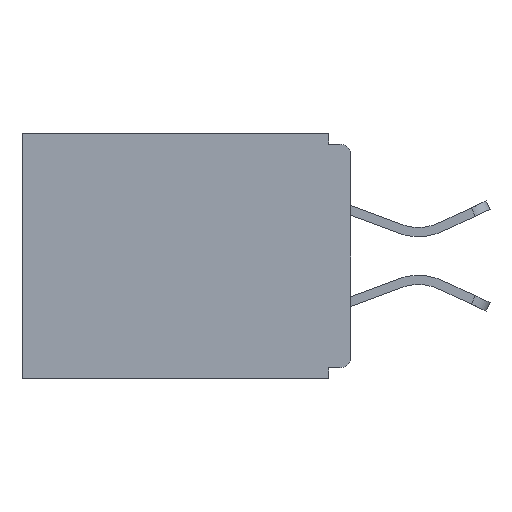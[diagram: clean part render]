
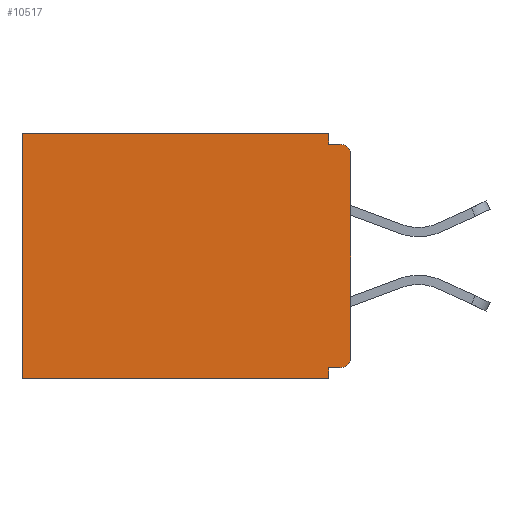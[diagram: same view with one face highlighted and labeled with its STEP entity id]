
A CAD part, left-side view. The second image highlights one B-rep face of the part: STEP entity #10517.
In plain terms, the highlighted planar face has unit normal (-1, 0, 0).
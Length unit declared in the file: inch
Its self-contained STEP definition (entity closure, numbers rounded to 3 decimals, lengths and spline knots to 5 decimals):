
#258 = ORIENTED_EDGE ( 'NONE', *, *, #4123, .F. ) ;
#387 = VERTEX_POINT ( 'NONE', #2516 ) ;
#434 = EDGE_CURVE ( 'NONE', #1373, #4286, #1137, .T. ) ;
#645 = DIRECTION ( 'NONE',  ( 0., 0., -1. ) ) ;
#848 = ORIENTED_EDGE ( 'NONE', *, *, #3834, .T. ) ;
#878 = CARTESIAN_POINT ( 'NONE',  ( 0.298, 0.015, -0.015 ) ) ;
#886 = VERTEX_POINT ( 'NONE', #5355 ) ;
#1010 = VECTOR ( 'NONE', #9738, 39.37008 ) ;
#1051 = ORIENTED_EDGE ( 'NONE', *, *, #8999, .T. ) ;
#1137 = LINE ( 'NONE', #3594, #8095 ) ;
#1141 = EDGE_CURVE ( 'NONE', #886, #8241, #9219, .T. ) ;
#1291 = LINE ( 'NONE', #1672, #3971 ) ;
#1373 = VERTEX_POINT ( 'NONE', #10183 ) ;
#1511 = CARTESIAN_POINT ( 'NONE',  ( 0.298, 0.031, -0.343 ) ) ;
#1668 = CARTESIAN_POINT ( 'NONE',  ( 0.298, 0.46, 0. ) ) ;
#1672 = CARTESIAN_POINT ( 'NONE',  ( 0.298, 0., -0.328 ) ) ;
#2212 = EDGE_CURVE ( 'NONE', #10403, #3517, #7458, .T. ) ;
#2218 = DIRECTION ( 'NONE',  ( 1., 0., 0. ) ) ;
#2272 = VERTEX_POINT ( 'NONE', #9874 ) ;
#2301 = LINE ( 'NONE', #1511, #4550 ) ;
#2417 = DIRECTION ( 'NONE',  ( 0., 1., 0. ) ) ;
#2439 = LINE ( 'NONE', #2885, #3441 ) ;
#2495 = CARTESIAN_POINT ( 'NONE',  ( 0.298, 0., 0. ) ) ;
#2516 = CARTESIAN_POINT ( 'NONE',  ( 0.298, 0.031, 0. ) ) ;
#2550 = CIRCLE ( 'NONE', #5939, 0.015 ) ;
#2885 = CARTESIAN_POINT ( 'NONE',  ( 0.298, 0.46, 0. ) ) ;
#3245 = CARTESIAN_POINT ( 'NONE',  ( 0.298, 0., 0. ) ) ;
#3380 = VECTOR ( 'NONE', #7256, 39.37008 ) ;
#3441 = VECTOR ( 'NONE', #6486, 39.37008 ) ;
#3517 = VERTEX_POINT ( 'NONE', #878 ) ;
#3594 = CARTESIAN_POINT ( 'NONE',  ( 0.298, 0., -0.343 ) ) ;
#3688 = ORIENTED_EDGE ( 'NONE', *, *, #434, .F. ) ;
#3762 = CARTESIAN_POINT ( 'NONE',  ( 0.298, 0.015, -0.328 ) ) ;
#3834 = EDGE_CURVE ( 'NONE', #7170, #4286, #2439, .T. ) ;
#3971 = VECTOR ( 'NONE', #2417, 39.37008 ) ;
#4009 = CARTESIAN_POINT ( 'NONE',  ( 0.298, 0.015, -0.03 ) ) ;
#4123 = EDGE_CURVE ( 'NONE', #2272, #1373, #2301, .T. ) ;
#4234 = DIRECTION ( 'NONE',  ( 0., 0., -1. ) ) ;
#4286 = VERTEX_POINT ( 'NONE', #5231 ) ;
#4450 = CARTESIAN_POINT ( 'NONE',  ( 0.298, 0.031, -0.343 ) ) ;
#4456 = ORIENTED_EDGE ( 'NONE', *, *, #10014, .T. ) ;
#4550 = VECTOR ( 'NONE', #4234, 39.37008 ) ;
#4786 = CIRCLE ( 'NONE', #5996, 0.015 ) ;
#5123 = VERTEX_POINT ( 'NONE', #3762 ) ;
#5131 = DIRECTION ( 'NONE',  ( -1., 0., 0. ) ) ;
#5165 = EDGE_CURVE ( 'NONE', #387, #10403, #5394, .T. ) ;
#5231 = CARTESIAN_POINT ( 'NONE',  ( 0.298, 0.46, -0.343 ) ) ;
#5355 = CARTESIAN_POINT ( 'NONE',  ( 0.298, 0., -0.03 ) ) ;
#5394 = LINE ( 'NONE', #4450, #9686 ) ;
#5908 = EDGE_CURVE ( 'NONE', #886, #3517, #2550, .T. ) ;
#5939 = AXIS2_PLACEMENT_3D ( 'NONE', #4009, #7741, #6828 ) ;
#5996 = AXIS2_PLACEMENT_3D ( 'NONE', #9586, #5131, #645 ) ;
#6379 = CARTESIAN_POINT ( 'NONE',  ( 0.298, 0., 0. ) ) ;
#6476 = EDGE_LOOP ( 'NONE', ( #10549, #10012, #6747, #1051, #848, #3688, #258, #8077, #4456, #6931 ) ) ;
#6486 = DIRECTION ( 'NONE',  ( 0., 0., -1. ) ) ;
#6747 = ORIENTED_EDGE ( 'NONE', *, *, #5165, .F. ) ;
#6828 = DIRECTION ( 'NONE',  ( 0., 0., -1. ) ) ;
#6931 = ORIENTED_EDGE ( 'NONE', *, *, #1141, .F. ) ;
#7170 = VERTEX_POINT ( 'NONE', #1668 ) ;
#7191 = DIRECTION ( 'NONE',  ( 0., -1., 0. ) ) ;
#7256 = DIRECTION ( 'NONE',  ( 0., 0., -1. ) ) ;
#7332 = CARTESIAN_POINT ( 'NONE',  ( 0.298, 0.031, -0.015 ) ) ;
#7458 = LINE ( 'NONE', #11454, #10459 ) ;
#7741 = DIRECTION ( 'NONE',  ( -1., 0., 0. ) ) ;
#7921 = FACE_OUTER_BOUND ( 'NONE', #6476, .T. ) ;
#8077 = ORIENTED_EDGE ( 'NONE', *, *, #9019, .F. ) ;
#8095 = VECTOR ( 'NONE', #9960, 39.37008 ) ;
#8241 = VERTEX_POINT ( 'NONE', #10516 ) ;
#8839 = AXIS2_PLACEMENT_3D ( 'NONE', #3245, #2218, #9535 ) ;
#8999 = EDGE_CURVE ( 'NONE', #387, #7170, #9253, .T. ) ;
#9019 = EDGE_CURVE ( 'NONE', #5123, #2272, #1291, .T. ) ;
#9097 = DIRECTION ( 'NONE',  ( 0., 0., -1. ) ) ;
#9219 = LINE ( 'NONE', #6379, #3380 ) ;
#9253 = LINE ( 'NONE', #2495, #1010 ) ;
#9535 = DIRECTION ( 'NONE',  ( 0., 0., -1. ) ) ;
#9586 = CARTESIAN_POINT ( 'NONE',  ( 0.298, 0.015, -0.313 ) ) ;
#9686 = VECTOR ( 'NONE', #9097, 39.37008 ) ;
#9738 = DIRECTION ( 'NONE',  ( 0., 1., 0. ) ) ;
#9874 = CARTESIAN_POINT ( 'NONE',  ( 0.298, 0.031, -0.328 ) ) ;
#9960 = DIRECTION ( 'NONE',  ( 0., 1., 0. ) ) ;
#10012 = ORIENTED_EDGE ( 'NONE', *, *, #2212, .F. ) ;
#10014 = EDGE_CURVE ( 'NONE', #5123, #8241, #4786, .T. ) ;
#10183 = CARTESIAN_POINT ( 'NONE',  ( 0.298, 0.031, -0.343 ) ) ;
#10403 = VERTEX_POINT ( 'NONE', #7332 ) ;
#10420 = PLANE ( 'NONE',  #8839 ) ;
#10459 = VECTOR ( 'NONE', #7191, 39.37008 ) ;
#10516 = CARTESIAN_POINT ( 'NONE',  ( 0.298, 0., -0.313 ) ) ;
#10517 = ADVANCED_FACE ( 'NONE', ( #7921 ), #10420, .F. ) ;
#10549 = ORIENTED_EDGE ( 'NONE', *, *, #5908, .T. ) ;
#11454 = CARTESIAN_POINT ( 'NONE',  ( 0.298, 0., -0.015 ) ) ;
